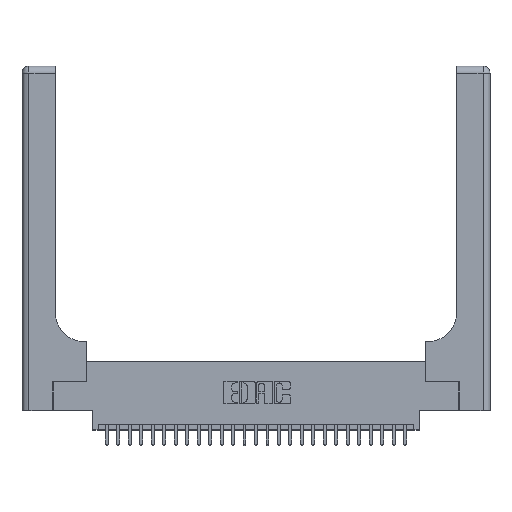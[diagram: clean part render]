
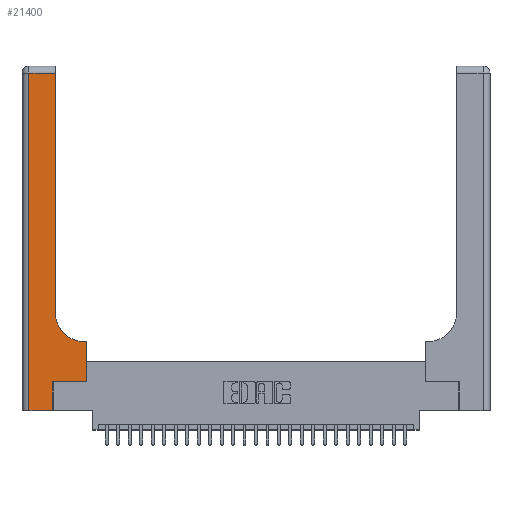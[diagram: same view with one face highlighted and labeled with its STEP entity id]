
A CAD part, top view. The second image highlights one B-rep face of the part: STEP entity #21400.
In plain terms, the highlighted planar face has unit normal (0, 0, 1).
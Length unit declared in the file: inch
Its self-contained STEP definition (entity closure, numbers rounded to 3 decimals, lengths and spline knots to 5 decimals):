
#594 = EDGE_CURVE ( 'NONE', #4597, #14879, #25541, .T. ) ;
#1067 = VERTEX_POINT ( 'NONE', #14807 ) ;
#1480 = LINE ( 'NONE', #19945, #25647 ) ;
#1560 = EDGE_CURVE ( 'NONE', #20205, #4597, #9792, .T. ) ;
#1671 = CARTESIAN_POINT ( 'NONE',  ( 0., 3., 0.37 ) ) ;
#1775 = DIRECTION ( 'NONE',  ( 0., 0., -1. ) ) ;
#1841 = ORIENTED_EDGE ( 'NONE', *, *, #11829, .T. ) ;
#2039 = CARTESIAN_POINT ( 'NONE',  ( 0.5415, 0.6, 0.37 ) ) ;
#2339 = DIRECTION ( 'NONE',  ( -1., 0., 0. ) ) ;
#2717 = VECTOR ( 'NONE', #7730, 39.37008 ) ;
#3103 = DIRECTION ( 'NONE',  ( -1., 0., 0. ) ) ;
#3580 = EDGE_LOOP ( 'NONE', ( #4630, #24687, #18156, #1841, #27435, #14232, #18293, #21436, #9953 ) ) ;
#3897 = DIRECTION ( 'NONE',  ( 1., 0., 0. ) ) ;
#3922 = DIRECTION ( 'NONE',  ( 0., 0., -1. ) ) ;
#3961 = CARTESIAN_POINT ( 'NONE',  ( 0.5415, 0.85, 0.37 ) ) ;
#3999 = VECTOR ( 'NONE', #7561, 39.37008 ) ;
#4597 = VERTEX_POINT ( 'NONE', #22313 ) ;
#4630 = ORIENTED_EDGE ( 'NONE', *, *, #594, .T. ) ;
#5545 = EDGE_CURVE ( 'NONE', #17710, #13915, #9920, .T. ) ;
#5939 = EDGE_CURVE ( 'NONE', #1067, #20205, #1480, .T. ) ;
#7561 = DIRECTION ( 'NONE',  ( 0., 1., 0. ) ) ;
#7730 = DIRECTION ( 'NONE',  ( 0., 1., 0. ) ) ;
#8445 = PLANE ( 'NONE',  #21663 ) ;
#9561 = LINE ( 'NONE', #17839, #20556 ) ;
#9792 = CIRCLE ( 'NONE', #14339, 0.25 ) ;
#9920 = LINE ( 'NONE', #22839, #3999 ) ;
#9953 = ORIENTED_EDGE ( 'NONE', *, *, #1560, .T. ) ;
#10381 = VERTEX_POINT ( 'NONE', #17082 ) ;
#10741 = VECTOR ( 'NONE', #3103, 39.37008 ) ;
#11829 = EDGE_CURVE ( 'NONE', #25155, #17710, #20749, .T. ) ;
#13915 = VERTEX_POINT ( 'NONE', #27541 ) ;
#14232 = ORIENTED_EDGE ( 'NONE', *, *, #20281, .T. ) ;
#14339 = AXIS2_PLACEMENT_3D ( 'NONE', #3961, #3922, #3897 ) ;
#14540 = LINE ( 'NONE', #25281, #2717 ) ;
#14807 = CARTESIAN_POINT ( 'NONE',  ( 0.5585, 0.6, 0.37 ) ) ;
#14879 = VERTEX_POINT ( 'NONE', #21896 ) ;
#15020 = FACE_OUTER_BOUND ( 'NONE', #3580, .T. ) ;
#15429 = CARTESIAN_POINT ( 'NONE',  ( 0.06, 3., 0.37 ) ) ;
#15758 = CARTESIAN_POINT ( 'NONE',  ( 0.06, 0., 0.37 ) ) ;
#16586 = LINE ( 'NONE', #22873, #10741 ) ;
#16856 = VERTEX_POINT ( 'NONE', #22347 ) ;
#17082 = CARTESIAN_POINT ( 'NONE',  ( 0.06, 2.94, 0.37 ) ) ;
#17299 = DIRECTION ( 'NONE',  ( -1., 0., 0. ) ) ;
#17681 = EDGE_CURVE ( 'NONE', #14879, #10381, #16586, .T. ) ;
#17710 = VERTEX_POINT ( 'NONE', #23055 ) ;
#17839 = CARTESIAN_POINT ( 'NONE',  ( 0.269, 0.25, 0.37 ) ) ;
#18156 = ORIENTED_EDGE ( 'NONE', *, *, #24660, .T. ) ;
#18293 = ORIENTED_EDGE ( 'NONE', *, *, #25352, .T. ) ;
#18668 = VECTOR ( 'NONE', #21909, 39.37008 ) ;
#19749 = DIRECTION ( 'NONE',  ( 1., 0., 0. ) ) ;
#19945 = CARTESIAN_POINT ( 'NONE',  ( 0.2915, 0.6, 0.37 ) ) ;
#20026 = DIRECTION ( 'NONE',  ( 1., 0., 0. ) ) ;
#20059 = VECTOR ( 'NONE', #19749, 39.37008 ) ;
#20205 = VERTEX_POINT ( 'NONE', #2039 ) ;
#20281 = EDGE_CURVE ( 'NONE', #13915, #16856, #9561, .T. ) ;
#20556 = VECTOR ( 'NONE', #20026, 39.37008 ) ;
#20749 = LINE ( 'NONE', #24143, #20059 ) ;
#21400 = ADVANCED_FACE ( 'NONE', ( #15020 ), #8445, .F. ) ;
#21436 = ORIENTED_EDGE ( 'NONE', *, *, #5939, .T. ) ;
#21663 = AXIS2_PLACEMENT_3D ( 'NONE', #1671, #1775, #17299 ) ;
#21896 = CARTESIAN_POINT ( 'NONE',  ( 0.2915, 2.94, 0.37 ) ) ;
#21909 = DIRECTION ( 'NONE',  ( 0., -1., 0. ) ) ;
#22313 = CARTESIAN_POINT ( 'NONE',  ( 0.2915, 0.85, 0.37 ) ) ;
#22347 = CARTESIAN_POINT ( 'NONE',  ( 0.5585, 0.25, 0.37 ) ) ;
#22429 = DIRECTION ( 'NONE',  ( 0., 1., 0. ) ) ;
#22620 = CARTESIAN_POINT ( 'NONE',  ( 0.2915, 3., 0.37 ) ) ;
#22839 = CARTESIAN_POINT ( 'NONE',  ( 0.269, 0., 0.37 ) ) ;
#22873 = CARTESIAN_POINT ( 'NONE',  ( 0., 2.94, 0.37 ) ) ;
#23055 = CARTESIAN_POINT ( 'NONE',  ( 0.269, 0., 0.37 ) ) ;
#24143 = CARTESIAN_POINT ( 'NONE',  ( 0., 0., 0.37 ) ) ;
#24479 = LINE ( 'NONE', #15429, #18668 ) ;
#24660 = EDGE_CURVE ( 'NONE', #10381, #25155, #24479, .T. ) ;
#24687 = ORIENTED_EDGE ( 'NONE', *, *, #17681, .T. ) ;
#24876 = VECTOR ( 'NONE', #22429, 39.37008 ) ;
#25155 = VERTEX_POINT ( 'NONE', #15758 ) ;
#25281 = CARTESIAN_POINT ( 'NONE',  ( 0.5585, 0.25, 0.37 ) ) ;
#25352 = EDGE_CURVE ( 'NONE', #16856, #1067, #14540, .T. ) ;
#25541 = LINE ( 'NONE', #22620, #24876 ) ;
#25647 = VECTOR ( 'NONE', #2339, 39.37008 ) ;
#27435 = ORIENTED_EDGE ( 'NONE', *, *, #5545, .T. ) ;
#27541 = CARTESIAN_POINT ( 'NONE',  ( 0.269, 0.25, 0.37 ) ) ;
